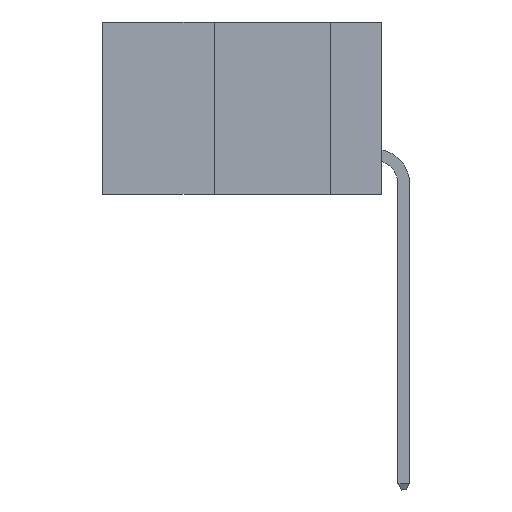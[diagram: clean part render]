
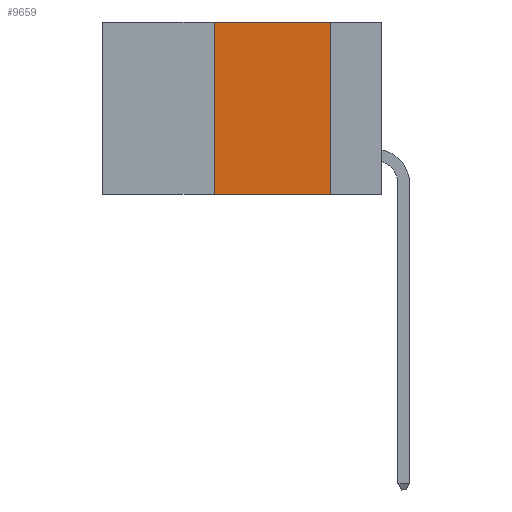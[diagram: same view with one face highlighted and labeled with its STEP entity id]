
A CAD part, left-side view. The second image highlights one B-rep face of the part: STEP entity #9659.
In plain terms, the highlighted planar face has unit normal (-1, 0, 0).
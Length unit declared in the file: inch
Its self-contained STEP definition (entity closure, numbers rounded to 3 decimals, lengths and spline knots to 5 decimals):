
#292 = LINE ( 'NONE', #9003, #4840 ) ;
#631 = CARTESIAN_POINT ( 'NONE',  ( 0., 0.6, 0. ) ) ;
#1293 = LINE ( 'NONE', #631, #8670 ) ;
#1499 = DIRECTION ( 'NONE',  ( 0., -1., 0. ) ) ;
#2027 = ORIENTED_EDGE ( 'NONE', *, *, #6250, .F. ) ;
#2503 = ORIENTED_EDGE ( 'NONE', *, *, #3001, .F. ) ;
#2861 = ORIENTED_EDGE ( 'NONE', *, *, #10790, .F. ) ;
#3001 = EDGE_CURVE ( 'NONE', #6981, #4992, #1293, .T. ) ;
#3085 = ORIENTED_EDGE ( 'NONE', *, *, #10636, .T. ) ;
#3549 = DIRECTION ( 'NONE',  ( 0., 0., -1. ) ) ;
#4389 = VECTOR ( 'NONE', #1499, 39.37008 ) ;
#4513 = VERTEX_POINT ( 'NONE', #9711 ) ;
#4840 = VECTOR ( 'NONE', #7400, 39.37008 ) ;
#4992 = VERTEX_POINT ( 'NONE', #7916 ) ;
#5139 = CARTESIAN_POINT ( 'NONE',  ( 0., 0.11, 0. ) ) ;
#5240 = FACE_OUTER_BOUND ( 'NONE', #9763, .T. ) ;
#5311 = LINE ( 'NONE', #5139, #7313 ) ;
#5369 = VERTEX_POINT ( 'NONE', #6539 ) ;
#6214 = CARTESIAN_POINT ( 'NONE',  ( 0., 0.6, 0. ) ) ;
#6250 = EDGE_CURVE ( 'NONE', #4992, #4513, #5311, .T. ) ;
#6539 = CARTESIAN_POINT ( 'NONE',  ( 0., 0.36, -0.37 ) ) ;
#6981 = VERTEX_POINT ( 'NONE', #11064 ) ;
#7005 = LINE ( 'NONE', #7797, #4389 ) ;
#7102 = DIRECTION ( 'NONE',  ( 0., -1., 0. ) ) ;
#7313 = VECTOR ( 'NONE', #10074, 39.37008 ) ;
#7400 = DIRECTION ( 'NONE',  ( 0., 0., 1. ) ) ;
#7797 = CARTESIAN_POINT ( 'NONE',  ( 0., 0.6, -0.37 ) ) ;
#7888 = PLANE ( 'NONE',  #11396 ) ;
#7916 = CARTESIAN_POINT ( 'NONE',  ( 0., 0.11, 0. ) ) ;
#8670 = VECTOR ( 'NONE', #7102, 39.37008 ) ;
#8685 = DIRECTION ( 'NONE',  ( 1., 0., 0. ) ) ;
#9003 = CARTESIAN_POINT ( 'NONE',  ( 0., 0.36, 0. ) ) ;
#9659 = ADVANCED_FACE ( 'NONE', ( #5240 ), #7888, .F. ) ;
#9711 = CARTESIAN_POINT ( 'NONE',  ( 0., 0.11, -0.37 ) ) ;
#9763 = EDGE_LOOP ( 'NONE', ( #2027, #2503, #2861, #3085 ) ) ;
#10074 = DIRECTION ( 'NONE',  ( 0., 0., -1. ) ) ;
#10636 = EDGE_CURVE ( 'NONE', #5369, #4513, #7005, .T. ) ;
#10790 = EDGE_CURVE ( 'NONE', #5369, #6981, #292, .T. ) ;
#11064 = CARTESIAN_POINT ( 'NONE',  ( 0., 0.36, 0. ) ) ;
#11396 = AXIS2_PLACEMENT_3D ( 'NONE', #6214, #8685, #3549 ) ;
